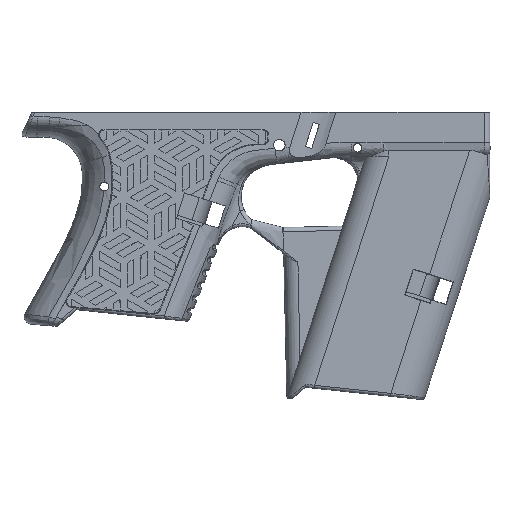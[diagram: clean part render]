
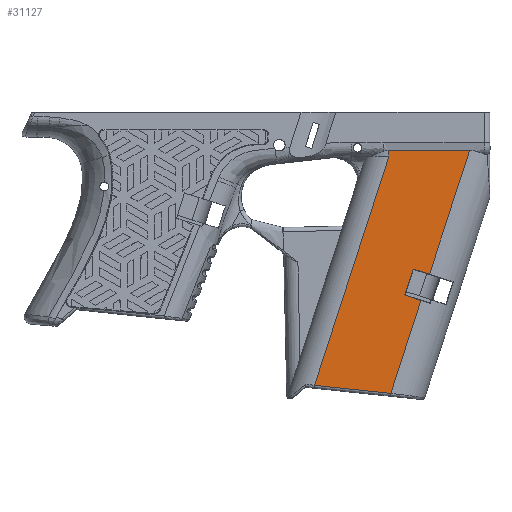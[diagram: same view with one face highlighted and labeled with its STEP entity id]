
A CAD part, top view. The second image highlights one B-rep face of the part: STEP entity #31127.
In plain terms, the highlighted planar face has unit normal (0, 0, 1).
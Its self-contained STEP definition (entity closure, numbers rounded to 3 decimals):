
#1715=PLANE('',#32739);
#3199=LINE('',#39769,#5865);
#3201=LINE('',#39781,#5867);
#3203=LINE('',#39793,#5869);
#3207=LINE('',#39935,#5873);
#3209=LINE('',#39964,#5875);
#4945=LINE('',#52050,#7611);
#4974=LINE('',#54941,#7640);
#5004=LINE('',#55535,#7670);
#5005=LINE('',#55536,#7671);
#5865=VECTOR('',#33695,10.);
#5867=VECTOR('',#33709,10.);
#5869=VECTOR('',#33723,10.);
#5873=VECTOR('',#33751,10.);
#5875=VECTOR('',#33759,10.);
#7611=VECTOR('',#36959,10.);
#7640=VECTOR('',#37108,10.);
#7670=VECTOR('',#37172,10.);
#7671=VECTOR('',#37173,10.);
#9766=FACE_OUTER_BOUND('',#11574,.T.);
#11574=EDGE_LOOP('',(#26198,#26199,#26200,#26201,#26202,#26203,#26204,#26205,
#26206,#26207,#26208));
#12330=CIRCLE('',#31906,0.2);
#12334=CIRCLE('',#31912,0.225);
#12878=VERTEX_POINT('',#39762);
#12880=VERTEX_POINT('',#39767);
#12882=VERTEX_POINT('',#39773);
#12884=VERTEX_POINT('',#39779);
#12886=VERTEX_POINT('',#39785);
#12888=VERTEX_POINT('',#39791);
#12897=VERTEX_POINT('',#39934);
#12903=VERTEX_POINT('',#39962);
#14649=VERTEX_POINT('',#52031);
#14757=VERTEX_POINT('',#54940);
#14793=VERTEX_POINT('',#55534);
#15937=EDGE_CURVE('',#12880,#12878,#3199,.T.);
#15940=EDGE_CURVE('',#12882,#12880,#12330,.T.);
#15943=EDGE_CURVE('',#12884,#12882,#3201,.T.);
#15946=EDGE_CURVE('',#12886,#12884,#12334,.T.);
#15949=EDGE_CURVE('',#12888,#12886,#3203,.T.);
#15965=EDGE_CURVE('',#12878,#12897,#3207,.T.);
#15972=EDGE_CURVE('',#12903,#12888,#3209,.T.);
#18634=EDGE_CURVE('',#12897,#14649,#4945,.T.);
#18779=EDGE_CURVE('',#14649,#14757,#4974,.T.);
#18836=EDGE_CURVE('',#14793,#12903,#5004,.T.);
#18837=EDGE_CURVE('',#14757,#14793,#5005,.T.);
#26198=ORIENTED_EDGE('',*,*,#15949,.F.);
#26199=ORIENTED_EDGE('',*,*,#15972,.F.);
#26200=ORIENTED_EDGE('',*,*,#18836,.F.);
#26201=ORIENTED_EDGE('',*,*,#18837,.F.);
#26202=ORIENTED_EDGE('',*,*,#18779,.F.);
#26203=ORIENTED_EDGE('',*,*,#18634,.F.);
#26204=ORIENTED_EDGE('',*,*,#15965,.F.);
#26205=ORIENTED_EDGE('',*,*,#15937,.F.);
#26206=ORIENTED_EDGE('',*,*,#15940,.F.);
#26207=ORIENTED_EDGE('',*,*,#15943,.F.);
#26208=ORIENTED_EDGE('',*,*,#15946,.F.);
#31127=ADVANCED_FACE('',(#9766),#1715,.T.);
#31906=AXIS2_PLACEMENT_3D('',#39775,#33701,#33702);
#31912=AXIS2_PLACEMENT_3D('',#39787,#33715,#33716);
#32739=AXIS2_PLACEMENT_3D('',#55533,#37170,#37171);
#33695=DIRECTION('',(0.951,-0.309,0.));
#33701=DIRECTION('center_axis',(0.,0.,
1.));
#33702=DIRECTION('ref_axis',(-0.891,-0.454,0.));
#33709=DIRECTION('',(-0.309,-0.951,0.));
#33715=DIRECTION('center_axis',(0.,0.,
1.));
#33716=DIRECTION('ref_axis',(-0.454,0.891,0.));
#33723=DIRECTION('',(-0.951,0.309,0.));
#33751=DIRECTION('',(-0.309,-0.951,0.));
#33759=DIRECTION('',(-0.309,-0.951,0.));
#36959=DIRECTION('',(-0.995,0.104,0.));
#37108=DIRECTION('',(0.309,0.951,0.));
#37170=DIRECTION('center_axis',(0.,0.,
1.));
#37171=DIRECTION('ref_axis',(1.,0.,0.));
#37172=DIRECTION('',(1.,0.,0.));
#37173=DIRECTION('',(0.,1.,0.));
#39762=CARTESIAN_POINT('',(131.781,-67.944,13.901));
#39767=CARTESIAN_POINT('',(126.195,-66.128,13.901));
#39769=CARTESIAN_POINT('',(127.942,-66.696,13.901));
#39773=CARTESIAN_POINT('',(126.066,-65.876,13.901));
#39775=CARTESIAN_POINT('Origin',(126.256,-65.938,13.901));
#39779=CARTESIAN_POINT('',(128.965,-56.954,13.901));
#39781=CARTESIAN_POINT('',(127.44,-61.647,13.901));
#39785=CARTESIAN_POINT('',(129.249,-56.809,13.901));
#39787=CARTESIAN_POINT('Origin',(129.179,-57.023,13.901));
#39791=CARTESIAN_POINT('',(134.812,-58.617,13.901));
#39793=CARTESIAN_POINT('',(131.305,-57.477,13.901));
#39934=CARTESIAN_POINT('',(121.006,-101.107,13.901));
#39935=CARTESIAN_POINT('',(126.517,-84.145,13.901));
#39962=CARTESIAN_POINT('',(149.149,-14.491,13.901));
#39964=CARTESIAN_POINT('',(126.517,-84.145,13.901));
#52031=CARTESIAN_POINT('',(93.807,-98.25,13.901));
#52050=CARTESIAN_POINT('',(103.922,-99.312,13.901));
#54940=CARTESIAN_POINT('',(120.372,-16.491,13.901));
#54941=CARTESIAN_POINT('',(111.726,-43.102,13.901));
#55533=CARTESIAN_POINT('Origin',(121.024,-64.241,13.901));
#55534=CARTESIAN_POINT('',(120.372,-14.491,13.901));
#55535=CARTESIAN_POINT('',(113.121,-14.491,13.901));
#55536=CARTESIAN_POINT('',(120.372,-16.491,13.901));
